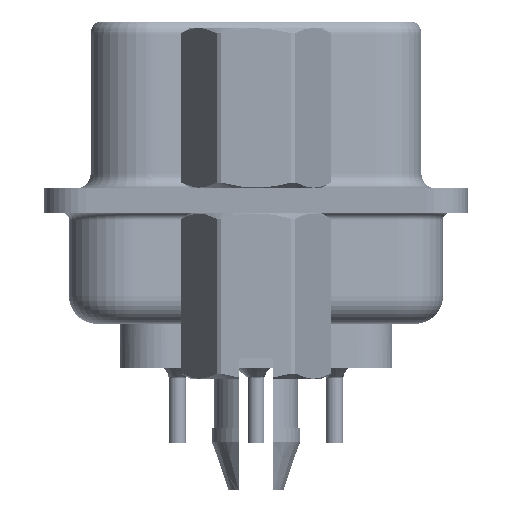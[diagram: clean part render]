
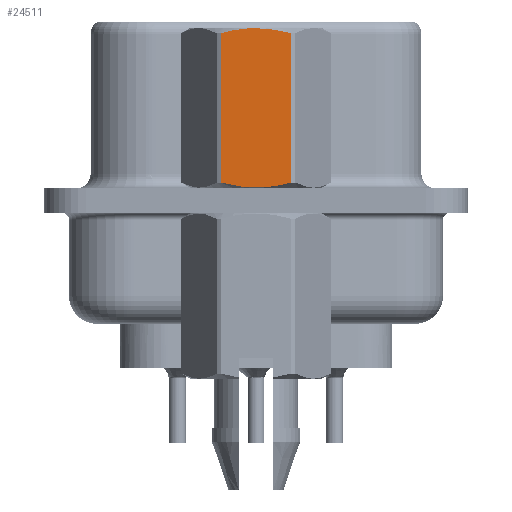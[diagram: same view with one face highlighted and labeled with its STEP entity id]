
A CAD part, left-side view. The second image highlights one B-rep face of the part: STEP entity #24511.
In plain terms, the highlighted planar face has unit normal (-1, 0, 0).
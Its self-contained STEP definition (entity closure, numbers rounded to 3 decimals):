
#1242 = PLANE ( 'NONE',  #32843 ) ;
#1385 = DIRECTION ( 'NONE',  ( -1., 0., 0. ) ) ;
#3250 = CARTESIAN_POINT ( 'NONE',  ( -2.381, 0.853, 6.151 ) ) ;
#3972 = FACE_OUTER_BOUND ( 'NONE', #25211, .T. ) ;
#4986 = LINE ( 'NONE', #32624, #21022 ) ;
#6413 = CARTESIAN_POINT ( 'NONE',  ( -2.381, -1.066, 6.104 ) ) ;
#6551 = CARTESIAN_POINT ( 'NONE',  ( -2.381, 1.273, 6.048 ) ) ;
#10347 = CARTESIAN_POINT ( 'NONE',  ( -2.381, 0.428, 0.485 ) ) ;
#11330 = ORIENTED_EDGE ( 'NONE', *, *, #15282, .T. ) ;
#11459 = VERTEX_POINT ( 'NONE', #23976 ) ;
#13537 = CARTESIAN_POINT ( 'NONE',  ( -2.381, -0.215, 0.468 ) ) ;
#15282 = EDGE_CURVE ( 'NONE', #16672, #23673, #4986, .T. ) ;
#16139 = CARTESIAN_POINT ( 'NONE',  ( -2.381, -0.858, 6.15 ) ) ;
#16672 = VERTEX_POINT ( 'NONE', #39078 ) ;
#16730 = CARTESIAN_POINT ( 'NONE',  ( -2.381, -0.858, 0.55 ) ) ;
#17028 = EDGE_CURVE ( 'NONE', #11459, #16672, #37607, .T. ) ;
#19154 = CARTESIAN_POINT ( 'NONE',  ( -2.381, -1.273, 6.048 ) ) ;
#19272 = CARTESIAN_POINT ( 'NONE',  ( -2.381, -0.215, 6.232 ) ) ;
#19866 = CARTESIAN_POINT ( 'NONE',  ( -2.381, -1.273, 0.652 ) ) ;
#20461 = VERTEX_POINT ( 'NONE', #23218 ) ;
#20705 = CARTESIAN_POINT ( 'NONE',  ( -2.381, 1.375, -3.75 ) ) ;
#21022 = VECTOR ( 'NONE', #23108, 1000. ) ;
#22480 = CARTESIAN_POINT ( 'NONE',  ( -2.381, 0.428, 6.215 ) ) ;
#23108 = DIRECTION ( 'NONE',  ( 0., 0., 1. ) ) ;
#23218 = CARTESIAN_POINT ( 'NONE',  ( -2.381, 1.273, 6.048 ) ) ;
#23455 = ORIENTED_EDGE ( 'NONE', *, *, #25635, .T. ) ;
#23638 = EDGE_CURVE ( 'NONE', #23673, #20461, #30907, .T. ) ;
#23673 = VERTEX_POINT ( 'NONE', #35169 ) ;
#23892 = DIRECTION ( 'NONE',  ( 0., -1., 0. ) ) ;
#23976 = CARTESIAN_POINT ( 'NONE',  ( -2.381, 1.273, 0.652 ) ) ;
#24511 = ADVANCED_FACE ( 'NONE', ( #3972 ), #1242, .T. ) ;
#25211 = EDGE_LOOP ( 'NONE', ( #37480, #11330, #39255, #23455 ) ) ;
#25622 = CARTESIAN_POINT ( 'NONE',  ( -2.381, 1.065, 6.104 ) ) ;
#25635 = EDGE_CURVE ( 'NONE', #20461, #11459, #26342, .T. ) ;
#26083 = DIRECTION ( 'NONE',  ( 0., 0., -1. ) ) ;
#26342 = LINE ( 'NONE', #38759, #33801 ) ;
#29091 = CARTESIAN_POINT ( 'NONE',  ( -2.381, 1.065, 0.596 ) ) ;
#29212 = CARTESIAN_POINT ( 'NONE',  ( -2.381, 0.853, 0.549 ) ) ;
#30907 = B_SPLINE_CURVE_WITH_KNOTS ( 'NONE', 3,
 ( #19154, #6413, #16139, #38251, #19272, #41473, #22480, #3250, #25622, #6551 ),
 .UNSPECIFIED., .F., .F.,
 ( 4, 2, 2, 2, 4 ),
 ( 0.001, 0.002, 0.002, 0.003, 0.004 ),
 .UNSPECIFIED. ) ;
#32468 = CARTESIAN_POINT ( 'NONE',  ( -2.381, 0.215, 0.468 ) ) ;
#32624 = CARTESIAN_POINT ( 'NONE',  ( -2.381, -1.273, 3.792 ) ) ;
#32843 = AXIS2_PLACEMENT_3D ( 'NONE', #20705, #1385, #23892 ) ;
#33801 = VECTOR ( 'NONE', #26083, 1000. ) ;
#35169 = CARTESIAN_POINT ( 'NONE',  ( -2.381, -1.273, 6.048 ) ) ;
#35632 = CARTESIAN_POINT ( 'NONE',  ( -2.381, -0.432, 0.485 ) ) ;
#37480 = ORIENTED_EDGE ( 'NONE', *, *, #17028, .T. ) ;
#37607 = B_SPLINE_CURVE_WITH_KNOTS ( 'NONE', 3,
 ( #38727, #29091, #29212, #10347, #32468, #13537, #35632, #16730, #38876, #19866 ),
 .UNSPECIFIED., .F., .F.,
 ( 4, 2, 2, 2, 4 ),
 ( 0.003, 0.003, 0.004, 0.004, 0.005 ),
 .UNSPECIFIED. ) ;
#38251 = CARTESIAN_POINT ( 'NONE',  ( -2.381, -0.432, 6.215 ) ) ;
#38727 = CARTESIAN_POINT ( 'NONE',  ( -2.381, 1.273, 0.652 ) ) ;
#38759 = CARTESIAN_POINT ( 'NONE',  ( -2.381, 1.273, 3.792 ) ) ;
#38876 = CARTESIAN_POINT ( 'NONE',  ( -2.381, -1.066, 0.596 ) ) ;
#39078 = CARTESIAN_POINT ( 'NONE',  ( -2.381, -1.273, 0.652 ) ) ;
#39255 = ORIENTED_EDGE ( 'NONE', *, *, #23638, .T. ) ;
#41473 = CARTESIAN_POINT ( 'NONE',  ( -2.381, 0.215, 6.232 ) ) ;
